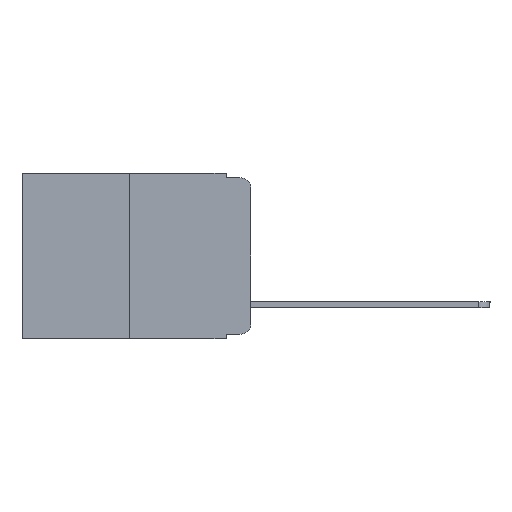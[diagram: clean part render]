
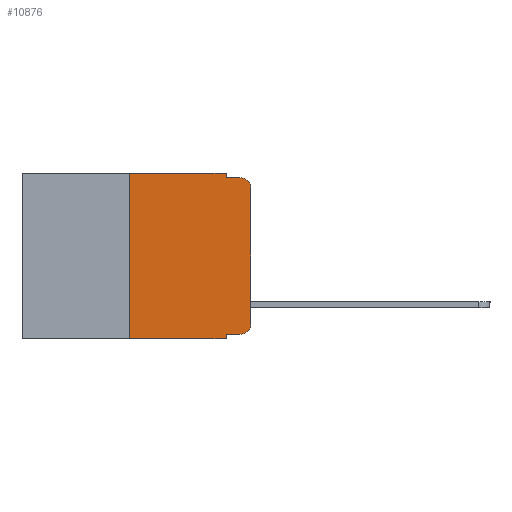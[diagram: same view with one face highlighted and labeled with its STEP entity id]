
A CAD part, left-side view. The second image highlights one B-rep face of the part: STEP entity #10876.
In plain terms, the highlighted planar face has unit normal (-1, 0, 0).
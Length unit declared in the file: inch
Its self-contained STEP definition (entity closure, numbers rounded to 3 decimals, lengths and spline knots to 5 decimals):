
#306 = LINE ( 'NONE', #17264, #10160 ) ;
#316 = VECTOR ( 'NONE', #18841, 39.37008 ) ;
#771 = ORIENTED_EDGE ( 'NONE', *, *, #5182, .F. ) ;
#1026 = CARTESIAN_POINT ( 'NONE',  ( 0., 0.473, -0.343 ) ) ;
#1477 = CIRCLE ( 'NONE', #5859, 0.02 ) ;
#1573 = DIRECTION ( 'NONE',  ( 0., 0., -1. ) ) ;
#2302 = CARTESIAN_POINT ( 'NONE',  ( 0., 0.473, 0. ) ) ;
#2417 = PLANE ( 'NONE',  #13772 ) ;
#2928 = DIRECTION ( 'NONE',  ( 0., 0., 1. ) ) ;
#3287 = FACE_OUTER_BOUND ( 'NONE', #6719, .T. ) ;
#4502 = EDGE_CURVE ( 'NONE', #22564, #7227, #22051, .T. ) ;
#5008 = EDGE_CURVE ( 'NONE', #17073, #5660, #5227, .T. ) ;
#5035 = CARTESIAN_POINT ( 'NONE',  ( 0., 0., 0. ) ) ;
#5182 = EDGE_CURVE ( 'NONE', #5660, #7741, #14109, .T. ) ;
#5227 = LINE ( 'NONE', #20841, #316 ) ;
#5660 = VERTEX_POINT ( 'NONE', #8441 ) ;
#5859 = AXIS2_PLACEMENT_3D ( 'NONE', #19897, #10398, #6288 ) ;
#5933 = CARTESIAN_POINT ( 'NONE',  ( 0., 0., -0.313 ) ) ;
#6164 = VECTOR ( 'NONE', #20405, 39.37008 ) ;
#6288 = DIRECTION ( 'NONE',  ( 0., 0., -1. ) ) ;
#6457 = VERTEX_POINT ( 'NONE', #19628 ) ;
#6541 = EDGE_CURVE ( 'NONE', #17073, #7227, #10129, .T. ) ;
#6719 = EDGE_LOOP ( 'NONE', ( #8926, #23280, #20918, #9179, #771, #17790, #12410, #8589, #12951, #17220 ) ) ;
#7019 = CARTESIAN_POINT ( 'NONE',  ( 0., 0.051, -0.01 ) ) ;
#7227 = VERTEX_POINT ( 'NONE', #19169 ) ;
#7250 = VERTEX_POINT ( 'NONE', #5933 ) ;
#7651 = DIRECTION ( 'NONE',  ( 0., 0., -1. ) ) ;
#7741 = VERTEX_POINT ( 'NONE', #15766 ) ;
#8032 = DIRECTION ( 'NONE',  ( 0., -1., 0. ) ) ;
#8441 = CARTESIAN_POINT ( 'NONE',  ( 0., 0.25, 0. ) ) ;
#8526 = LINE ( 'NONE', #5035, #13776 ) ;
#8589 = ORIENTED_EDGE ( 'NONE', *, *, #4502, .F. ) ;
#8637 = DIRECTION ( 'NONE',  ( 0., -1., 0. ) ) ;
#8926 = ORIENTED_EDGE ( 'NONE', *, *, #9248, .T. ) ;
#9009 = EDGE_CURVE ( 'NONE', #7741, #23196, #24685, .T. ) ;
#9179 = ORIENTED_EDGE ( 'NONE', *, *, #9009, .F. ) ;
#9248 = EDGE_CURVE ( 'NONE', #7250, #12498, #8526, .T. ) ;
#10024 = EDGE_CURVE ( 'NONE', #22564, #19769, #22993, .T. ) ;
#10129 = LINE ( 'NONE', #1026, #19511 ) ;
#10160 = VECTOR ( 'NONE', #8032, 39.37008 ) ;
#10398 = DIRECTION ( 'NONE',  ( -1., 0., 0. ) ) ;
#10754 = CARTESIAN_POINT ( 'NONE',  ( 0., 0.25, -0.343 ) ) ;
#10876 = ADVANCED_FACE ( 'NONE', ( #3287 ), #2417, .F. ) ;
#11766 = DIRECTION ( 'NONE',  ( 1., 0., 0. ) ) ;
#12410 = ORIENTED_EDGE ( 'NONE', *, *, #6541, .T. ) ;
#12498 = VERTEX_POINT ( 'NONE', #21504 ) ;
#12776 = EDGE_CURVE ( 'NONE', #12498, #6457, #19846, .T. ) ;
#12951 = ORIENTED_EDGE ( 'NONE', *, *, #10024, .T. ) ;
#13772 = AXIS2_PLACEMENT_3D ( 'NONE', #2302, #11766, #7651 ) ;
#13776 = VECTOR ( 'NONE', #2928, 39.37008 ) ;
#14109 = LINE ( 'NONE', #22083, #20647 ) ;
#15041 = EDGE_CURVE ( 'NONE', #23196, #6457, #306, .T. ) ;
#15766 = CARTESIAN_POINT ( 'NONE',  ( 0., 0.051, 0. ) ) ;
#15979 = DIRECTION ( 'NONE',  ( 0., -1., 0. ) ) ;
#16453 = CARTESIAN_POINT ( 'NONE',  ( 0., 0.02, -0.03 ) ) ;
#16985 = EDGE_CURVE ( 'NONE', #19769, #7250, #1477, .T. ) ;
#17073 = VERTEX_POINT ( 'NONE', #10754 ) ;
#17220 = ORIENTED_EDGE ( 'NONE', *, *, #16985, .T. ) ;
#17264 = CARTESIAN_POINT ( 'NONE',  ( 0., 0.051, -0.01 ) ) ;
#17295 = VECTOR ( 'NONE', #17347, 39.37008 ) ;
#17347 = DIRECTION ( 'NONE',  ( 0., -1., 0. ) ) ;
#17437 = AXIS2_PLACEMENT_3D ( 'NONE', #16453, #24350, #22588 ) ;
#17790 = ORIENTED_EDGE ( 'NONE', *, *, #5008, .F. ) ;
#18646 = CARTESIAN_POINT ( 'NONE',  ( 0., 0.02, -0.333 ) ) ;
#18658 = CARTESIAN_POINT ( 'NONE',  ( 0., 0.051, 0. ) ) ;
#18787 = CARTESIAN_POINT ( 'NONE',  ( 0., 0.051, 0. ) ) ;
#18841 = DIRECTION ( 'NONE',  ( 0., 0., 1. ) ) ;
#19169 = CARTESIAN_POINT ( 'NONE',  ( 0., 0.051, -0.343 ) ) ;
#19443 = CARTESIAN_POINT ( 'NONE',  ( 0., 0.051, -0.333 ) ) ;
#19491 = CARTESIAN_POINT ( 'NONE',  ( 0., 0.051, -0.333 ) ) ;
#19511 = VECTOR ( 'NONE', #8637, 39.37008 ) ;
#19628 = CARTESIAN_POINT ( 'NONE',  ( 0., 0.02, -0.01 ) ) ;
#19769 = VERTEX_POINT ( 'NONE', #18646 ) ;
#19846 = CIRCLE ( 'NONE', #17437, 0.02 ) ;
#19897 = CARTESIAN_POINT ( 'NONE',  ( 0., 0.02, -0.313 ) ) ;
#20405 = DIRECTION ( 'NONE',  ( 0., 0., -1. ) ) ;
#20647 = VECTOR ( 'NONE', #15979, 39.37008 ) ;
#20841 = CARTESIAN_POINT ( 'NONE',  ( 0., 0.25, 0. ) ) ;
#20918 = ORIENTED_EDGE ( 'NONE', *, *, #15041, .F. ) ;
#21504 = CARTESIAN_POINT ( 'NONE',  ( 0., 0., -0.03 ) ) ;
#21855 = VECTOR ( 'NONE', #1573, 39.37008 ) ;
#22051 = LINE ( 'NONE', #18658, #21855 ) ;
#22083 = CARTESIAN_POINT ( 'NONE',  ( 0., 0.473, 0. ) ) ;
#22564 = VERTEX_POINT ( 'NONE', #19443 ) ;
#22588 = DIRECTION ( 'NONE',  ( 0., 0., -1. ) ) ;
#22993 = LINE ( 'NONE', #19491, #17295 ) ;
#23196 = VERTEX_POINT ( 'NONE', #7019 ) ;
#23280 = ORIENTED_EDGE ( 'NONE', *, *, #12776, .T. ) ;
#24350 = DIRECTION ( 'NONE',  ( -1., 0., 0. ) ) ;
#24685 = LINE ( 'NONE', #18787, #6164 ) ;
